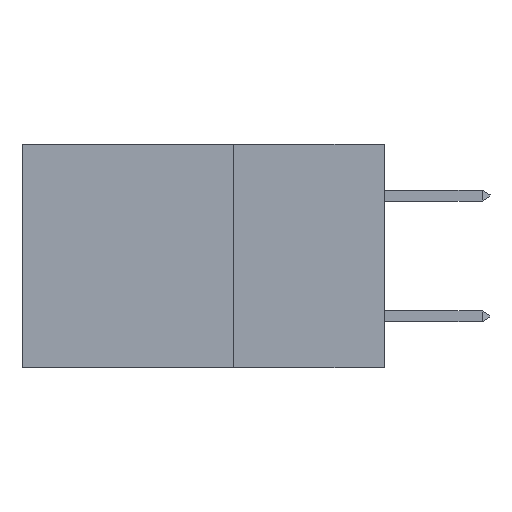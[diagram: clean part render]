
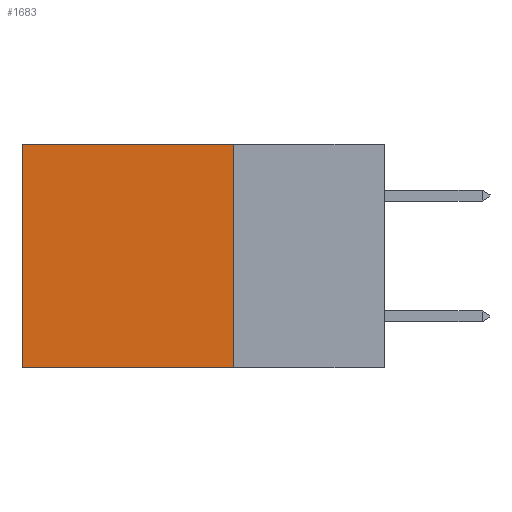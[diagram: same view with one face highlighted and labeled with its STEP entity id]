
A CAD part, left-side view. The second image highlights one B-rep face of the part: STEP entity #1683.
In plain terms, the highlighted planar face has unit normal (-1, 0, 0).
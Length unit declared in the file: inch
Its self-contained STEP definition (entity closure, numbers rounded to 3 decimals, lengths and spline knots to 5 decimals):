
#176 = VECTOR ( 'NONE', #7143, 39.37008 ) ;
#890 = ORIENTED_EDGE ( 'NONE', *, *, #10633, .T. ) ;
#985 = CARTESIAN_POINT ( 'NONE',  ( 0.2875, 0.25, 0. ) ) ;
#1683 = ADVANCED_FACE ( 'NONE', ( #1759 ), #11348, .F. ) ;
#1759 = FACE_OUTER_BOUND ( 'NONE', #10275, .T. ) ;
#2104 = VERTEX_POINT ( 'NONE', #985 ) ;
#2176 = DIRECTION ( 'NONE',  ( 0., 0., -1. ) ) ;
#2991 = CARTESIAN_POINT ( 'NONE',  ( 0.2875, 0.25, 0. ) ) ;
#3837 = CARTESIAN_POINT ( 'NONE',  ( 0.2875, 0.6, 0. ) ) ;
#4024 = EDGE_CURVE ( 'NONE', #2104, #8427, #13335, .T. ) ;
#4331 = DIRECTION ( 'NONE',  ( 0., 1., 0. ) ) ;
#4499 = VECTOR ( 'NONE', #4331, 39.37008 ) ;
#4821 = LINE ( 'NONE', #12503, #7521 ) ;
#5860 = ORIENTED_EDGE ( 'NONE', *, *, #12993, .T. ) ;
#6270 = VERTEX_POINT ( 'NONE', #3837 ) ;
#6492 = VERTEX_POINT ( 'NONE', #7535 ) ;
#6857 = CARTESIAN_POINT ( 'NONE',  ( 0.2875, 0.25, 0. ) ) ;
#7002 = ORIENTED_EDGE ( 'NONE', *, *, #4024, .F. ) ;
#7143 = DIRECTION ( 'NONE',  ( 0., 0., -1. ) ) ;
#7459 = VECTOR ( 'NONE', #2176, 39.37008 ) ;
#7521 = VECTOR ( 'NONE', #13507, 39.37008 ) ;
#7535 = CARTESIAN_POINT ( 'NONE',  ( 0.2875, 0.6, -0.37 ) ) ;
#8213 = DIRECTION ( 'NONE',  ( 0., 0., -1. ) ) ;
#8427 = VERTEX_POINT ( 'NONE', #8487 ) ;
#8487 = CARTESIAN_POINT ( 'NONE',  ( 0.2875, 0.25, -0.37 ) ) ;
#8991 = CARTESIAN_POINT ( 'NONE',  ( 0.2875, 0.25, -0.37 ) ) ;
#10275 = EDGE_LOOP ( 'NONE', ( #5860, #11745, #7002, #890 ) ) ;
#10571 = CARTESIAN_POINT ( 'NONE',  ( 0.2875, 0.6, 0. ) ) ;
#10581 = LINE ( 'NONE', #8991, #4499 ) ;
#10633 = EDGE_CURVE ( 'NONE', #2104, #6270, #4821, .T. ) ;
#11348 = PLANE ( 'NONE',  #14528 ) ;
#11745 = ORIENTED_EDGE ( 'NONE', *, *, #12738, .F. ) ;
#12503 = CARTESIAN_POINT ( 'NONE',  ( 0.2875, 0.25, 0. ) ) ;
#12657 = LINE ( 'NONE', #10571, #176 ) ;
#12738 = EDGE_CURVE ( 'NONE', #8427, #6492, #10581, .T. ) ;
#12993 = EDGE_CURVE ( 'NONE', #6270, #6492, #12657, .T. ) ;
#13335 = LINE ( 'NONE', #2991, #7459 ) ;
#13507 = DIRECTION ( 'NONE',  ( 0., 1., 0. ) ) ;
#14063 = DIRECTION ( 'NONE',  ( 1., 0., 0. ) ) ;
#14528 = AXIS2_PLACEMENT_3D ( 'NONE', #6857, #14063, #8213 ) ;
